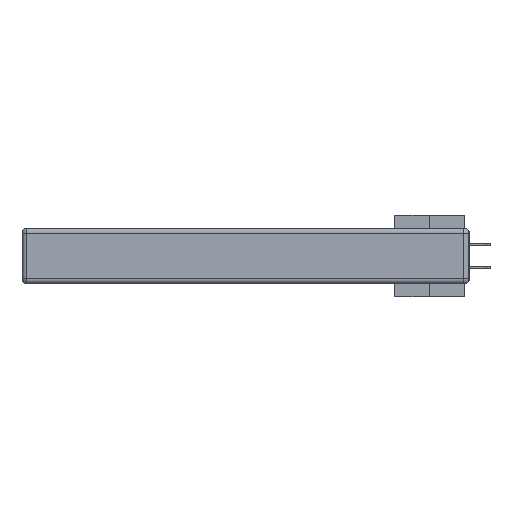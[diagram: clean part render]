
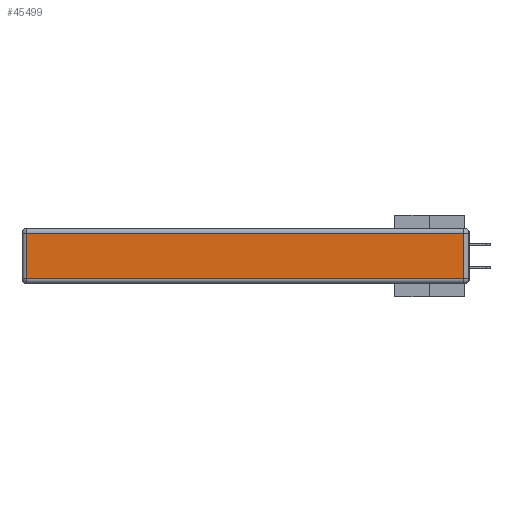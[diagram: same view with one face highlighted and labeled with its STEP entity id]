
A CAD part, left-side view. The second image highlights one B-rep face of the part: STEP entity #45499.
In plain terms, the highlighted planar face has unit normal (-1, 0, 0).
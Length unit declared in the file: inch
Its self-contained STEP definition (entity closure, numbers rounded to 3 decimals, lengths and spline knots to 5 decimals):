
#502 = CARTESIAN_POINT ( 'NONE',  ( 0., 2.72, -0.343 ) ) ;
#1295 = LINE ( 'NONE', #5644, #10007 ) ;
#2456 = CARTESIAN_POINT ( 'NONE',  ( 0., 0.03, -0.343 ) ) ;
#2690 = CARTESIAN_POINT ( 'NONE',  ( 0., 2.72, -0.03 ) ) ;
#5644 = CARTESIAN_POINT ( 'NONE',  ( 0., 2.75, -0.03 ) ) ;
#8584 = VECTOR ( 'NONE', #20291, 39.37008 ) ;
#9779 = LINE ( 'NONE', #502, #40601 ) ;
#10007 = VECTOR ( 'NONE', #20727, 39.37008 ) ;
#10431 = FACE_OUTER_BOUND ( 'NONE', #44422, .T. ) ;
#11256 = LINE ( 'NONE', #28311, #43236 ) ;
#12023 = AXIS2_PLACEMENT_3D ( 'NONE', #12562, #16122, #38176 ) ;
#12562 = CARTESIAN_POINT ( 'NONE',  ( 0., 0., -0.343 ) ) ;
#12972 = CARTESIAN_POINT ( 'NONE',  ( 0., 0.03, -0.313 ) ) ;
#13023 = ORIENTED_EDGE ( 'NONE', *, *, #45961, .T. ) ;
#15356 = CARTESIAN_POINT ( 'NONE',  ( 0., 0.03, -0.03 ) ) ;
#16122 = DIRECTION ( 'NONE',  ( -1., 0., 0. ) ) ;
#19819 = PLANE ( 'NONE',  #12023 ) ;
#20291 = DIRECTION ( 'NONE',  ( 0., 0., 1. ) ) ;
#20727 = DIRECTION ( 'NONE',  ( 0., 1., 0. ) ) ;
#23896 = VERTEX_POINT ( 'NONE', #2690 ) ;
#24733 = EDGE_CURVE ( 'NONE', #30225, #23896, #1295, .T. ) ;
#27549 = ORIENTED_EDGE ( 'NONE', *, *, #34295, .T. ) ;
#27583 = EDGE_CURVE ( 'NONE', #23896, #31010, #9779, .T. ) ;
#28311 = CARTESIAN_POINT ( 'NONE',  ( 0., 0., -0.313 ) ) ;
#30225 = VERTEX_POINT ( 'NONE', #15356 ) ;
#31010 = VERTEX_POINT ( 'NONE', #44918 ) ;
#34295 = EDGE_CURVE ( 'NONE', #31010, #39991, #11256, .T. ) ;
#35289 = DIRECTION ( 'NONE',  ( 0., -1., 0. ) ) ;
#36689 = ORIENTED_EDGE ( 'NONE', *, *, #27583, .T. ) ;
#37464 = DIRECTION ( 'NONE',  ( 0., 0., -1. ) ) ;
#37619 = LINE ( 'NONE', #2456, #8584 ) ;
#38176 = DIRECTION ( 'NONE',  ( 0., 0., 1. ) ) ;
#39991 = VERTEX_POINT ( 'NONE', #12972 ) ;
#40601 = VECTOR ( 'NONE', #37464, 39.37008 ) ;
#43236 = VECTOR ( 'NONE', #35289, 39.37008 ) ;
#44422 = EDGE_LOOP ( 'NONE', ( #27549, #13023, #47472, #36689 ) ) ;
#44918 = CARTESIAN_POINT ( 'NONE',  ( 0., 2.72, -0.313 ) ) ;
#45499 = ADVANCED_FACE ( 'NONE', ( #10431 ), #19819, .T. ) ;
#45961 = EDGE_CURVE ( 'NONE', #39991, #30225, #37619, .T. ) ;
#47472 = ORIENTED_EDGE ( 'NONE', *, *, #24733, .T. ) ;
